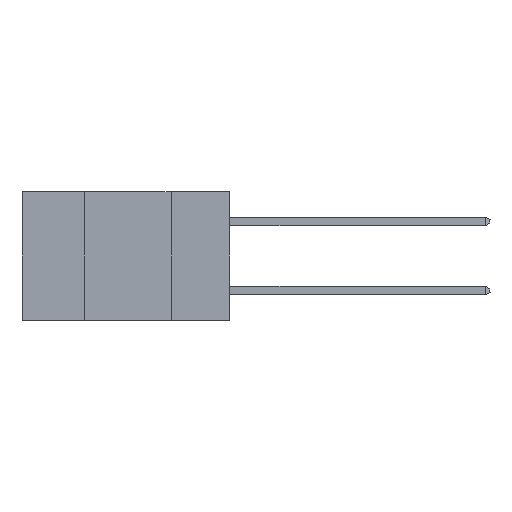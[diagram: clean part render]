
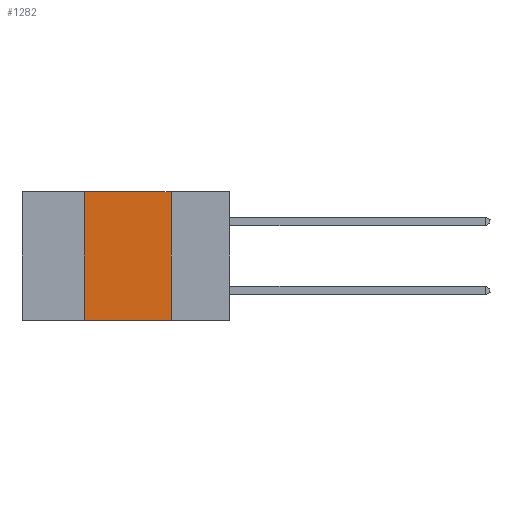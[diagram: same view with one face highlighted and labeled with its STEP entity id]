
A CAD part, left-side view. The second image highlights one B-rep face of the part: STEP entity #1282.
In plain terms, the highlighted planar face has unit normal (-1, 0, 0).
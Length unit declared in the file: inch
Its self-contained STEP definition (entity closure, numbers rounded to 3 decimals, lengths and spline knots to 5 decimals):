
#324 = DIRECTION ( 'NONE',  ( 0., 0., -1. ) ) ;
#476 = DIRECTION ( 'NONE',  ( 0., -1., 0. ) ) ;
#674 = LINE ( 'NONE', #21745, #9040 ) ;
#1023 = AXIS2_PLACEMENT_3D ( 'NONE', #10523, #5477, #19103 ) ;
#1115 = DIRECTION ( 'NONE',  ( 0., -1., 0. ) ) ;
#1282 = ADVANCED_FACE ( 'NONE', ( #5717 ), #11647, .F. ) ;
#1637 = CARTESIAN_POINT ( 'NONE',  ( 0., 0.17, -0.37 ) ) ;
#1701 = DIRECTION ( 'NONE',  ( 0., 0., 1. ) ) ;
#3241 = VERTEX_POINT ( 'NONE', #9470 ) ;
#3560 = CARTESIAN_POINT ( 'NONE',  ( 0., 0.17, 0. ) ) ;
#3947 = VERTEX_POINT ( 'NONE', #1637 ) ;
#4252 = VECTOR ( 'NONE', #1701, 39.37008 ) ;
#5477 = DIRECTION ( 'NONE',  ( 1., 0., 0. ) ) ;
#5717 = FACE_OUTER_BOUND ( 'NONE', #13650, .T. ) ;
#6816 = VECTOR ( 'NONE', #476, 39.37008 ) ;
#7047 = ORIENTED_EDGE ( 'NONE', *, *, #13094, .F. ) ;
#8731 = ORIENTED_EDGE ( 'NONE', *, *, #12273, .F. ) ;
#8922 = ORIENTED_EDGE ( 'NONE', *, *, #21935, .F. ) ;
#9040 = VECTOR ( 'NONE', #1115, 39.37008 ) ;
#9470 = CARTESIAN_POINT ( 'NONE',  ( 0., 0.17, 0. ) ) ;
#9924 = VERTEX_POINT ( 'NONE', #19377 ) ;
#10523 = CARTESIAN_POINT ( 'NONE',  ( 0., 0.6, 0. ) ) ;
#11179 = VERTEX_POINT ( 'NONE', #16784 ) ;
#11647 = PLANE ( 'NONE',  #1023 ) ;
#12273 = EDGE_CURVE ( 'NONE', #11179, #3241, #13511, .T. ) ;
#12396 = LINE ( 'NONE', #3560, #15917 ) ;
#12410 = CARTESIAN_POINT ( 'NONE',  ( 0., 0.6, 0. ) ) ;
#13094 = EDGE_CURVE ( 'NONE', #3241, #3947, #12396, .T. ) ;
#13309 = ORIENTED_EDGE ( 'NONE', *, *, #15368, .T. ) ;
#13511 = LINE ( 'NONE', #12410, #6816 ) ;
#13650 = EDGE_LOOP ( 'NONE', ( #7047, #8731, #8922, #13309 ) ) ;
#13671 = LINE ( 'NONE', #15369, #4252 ) ;
#15368 = EDGE_CURVE ( 'NONE', #9924, #3947, #674, .T. ) ;
#15369 = CARTESIAN_POINT ( 'NONE',  ( 0., 0.42, 0. ) ) ;
#15917 = VECTOR ( 'NONE', #324, 39.37008 ) ;
#16784 = CARTESIAN_POINT ( 'NONE',  ( 0., 0.42, 0. ) ) ;
#19103 = DIRECTION ( 'NONE',  ( 0., 0., -1. ) ) ;
#19377 = CARTESIAN_POINT ( 'NONE',  ( 0., 0.42, -0.37 ) ) ;
#21745 = CARTESIAN_POINT ( 'NONE',  ( 0., 0.6, -0.37 ) ) ;
#21935 = EDGE_CURVE ( 'NONE', #9924, #11179, #13671, .T. ) ;
